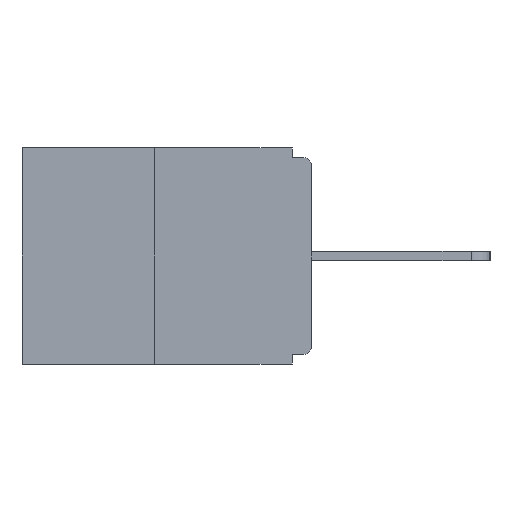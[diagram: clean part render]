
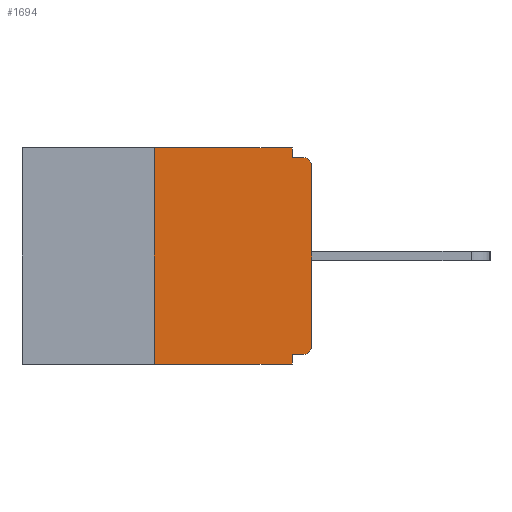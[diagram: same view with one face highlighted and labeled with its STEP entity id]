
A CAD part, left-side view. The second image highlights one B-rep face of the part: STEP entity #1694.
In plain terms, the highlighted planar face has unit normal (-1, 0, 0).
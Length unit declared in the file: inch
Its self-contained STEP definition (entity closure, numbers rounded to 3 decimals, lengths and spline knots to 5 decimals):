
#20 = CARTESIAN_POINT ( 'NONE',  ( 0., 0.46, 0. ) ) ;
#141 = CARTESIAN_POINT ( 'NONE',  ( 0., 0.015, -0.015 ) ) ;
#284 = CARTESIAN_POINT ( 'NONE',  ( 0., 0.031, 0. ) ) ;
#292 = LINE ( 'NONE', #13787, #13324 ) ;
#404 = EDGE_CURVE ( 'NONE', #16049, #15028, #6335, .T. ) ;
#788 = VERTEX_POINT ( 'NONE', #22123 ) ;
#1146 = VERTEX_POINT ( 'NONE', #5849 ) ;
#1694 = ADVANCED_FACE ( 'NONE', ( #17215 ), #3090, .F. ) ;
#1705 = VERTEX_POINT ( 'NONE', #16622 ) ;
#1894 = DIRECTION ( 'NONE',  ( 0., 0., -1. ) ) ;
#1922 = DIRECTION ( 'NONE',  ( -1., 0., 0. ) ) ;
#1966 = CARTESIAN_POINT ( 'NONE',  ( 0., 0.015, -0.03 ) ) ;
#2034 = EDGE_LOOP ( 'NONE', ( #8245, #4088, #13419, #9899, #2703, #16720, #3263, #17258, #22466, #19422 ) ) ;
#2648 = VERTEX_POINT ( 'NONE', #16496 ) ;
#2703 = ORIENTED_EDGE ( 'NONE', *, *, #9752, .F. ) ;
#3090 = PLANE ( 'NONE',  #18814 ) ;
#3263 = ORIENTED_EDGE ( 'NONE', *, *, #7796, .T. ) ;
#3947 = CARTESIAN_POINT ( 'NONE',  ( 0., 0., 0. ) ) ;
#3975 = DIRECTION ( 'NONE',  ( 0., 0., 1. ) ) ;
#4088 = ORIENTED_EDGE ( 'NONE', *, *, #10374, .F. ) ;
#4287 = VERTEX_POINT ( 'NONE', #141 ) ;
#4296 = LINE ( 'NONE', #3947, #18491 ) ;
#5050 = DIRECTION ( 'NONE',  ( 0., 0., -1. ) ) ;
#5373 = VECTOR ( 'NONE', #11786, 39.37008 ) ;
#5708 = CARTESIAN_POINT ( 'NONE',  ( 0., 0., -0.313 ) ) ;
#5849 = CARTESIAN_POINT ( 'NONE',  ( 0., 0.25, 0. ) ) ;
#5916 = LINE ( 'NONE', #10039, #5373 ) ;
#6121 = CARTESIAN_POINT ( 'NONE',  ( 0., 0., -0.015 ) ) ;
#6335 = CIRCLE ( 'NONE', #11204, 0.015 ) ;
#6812 = LINE ( 'NONE', #12746, #19632 ) ;
#6883 = LINE ( 'NONE', #20, #20272 ) ;
#7126 = VERTEX_POINT ( 'NONE', #11226 ) ;
#7226 = DIRECTION ( 'NONE',  ( -1., 0., 0. ) ) ;
#7796 = EDGE_CURVE ( 'NONE', #15028, #2648, #4296, .T. ) ;
#7945 = EDGE_CURVE ( 'NONE', #2648, #4287, #10362, .T. ) ;
#8245 = ORIENTED_EDGE ( 'NONE', *, *, #21274, .F. ) ;
#9752 = EDGE_CURVE ( 'NONE', #16049, #788, #6812, .T. ) ;
#9899 = ORIENTED_EDGE ( 'NONE', *, *, #10692, .F. ) ;
#10039 = CARTESIAN_POINT ( 'NONE',  ( 0., 0.031, 0. ) ) ;
#10362 = CIRCLE ( 'NONE', #14993, 0.015 ) ;
#10374 = EDGE_CURVE ( 'NONE', #1705, #1146, #16380, .T. ) ;
#10436 = VERTEX_POINT ( 'NONE', #18266 ) ;
#10692 = EDGE_CURVE ( 'NONE', #788, #10436, #292, .T. ) ;
#10855 = EDGE_CURVE ( 'NONE', #16241, #7126, #5916, .T. ) ;
#11204 = AXIS2_PLACEMENT_3D ( 'NONE', #16271, #7226, #11747 ) ;
#11226 = CARTESIAN_POINT ( 'NONE',  ( 0., 0.031, -0.015 ) ) ;
#11747 = DIRECTION ( 'NONE',  ( 0., 0., -1. ) ) ;
#11786 = DIRECTION ( 'NONE',  ( 0., 0., -1. ) ) ;
#12746 = CARTESIAN_POINT ( 'NONE',  ( 0., 0., -0.328 ) ) ;
#12875 = EDGE_CURVE ( 'NONE', #1705, #10436, #13781, .T. ) ;
#13324 = VECTOR ( 'NONE', #5050, 39.37008 ) ;
#13419 = ORIENTED_EDGE ( 'NONE', *, *, #12875, .T. ) ;
#13570 = VECTOR ( 'NONE', #16618, 39.37008 ) ;
#13781 = LINE ( 'NONE', #21096, #17857 ) ;
#13787 = CARTESIAN_POINT ( 'NONE',  ( 0., 0.031, -0.343 ) ) ;
#14516 = DIRECTION ( 'NONE',  ( 0., 1., 0. ) ) ;
#14660 = CARTESIAN_POINT ( 'NONE',  ( 0., 0.25, 0. ) ) ;
#14993 = AXIS2_PLACEMENT_3D ( 'NONE', #1966, #1922, #1894 ) ;
#15028 = VERTEX_POINT ( 'NONE', #5708 ) ;
#15846 = VECTOR ( 'NONE', #16414, 39.37008 ) ;
#16049 = VERTEX_POINT ( 'NONE', #22650 ) ;
#16241 = VERTEX_POINT ( 'NONE', #284 ) ;
#16271 = CARTESIAN_POINT ( 'NONE',  ( 0., 0.015, -0.313 ) ) ;
#16380 = LINE ( 'NONE', #14660, #15846 ) ;
#16414 = DIRECTION ( 'NONE',  ( 0., 0., 1. ) ) ;
#16496 = CARTESIAN_POINT ( 'NONE',  ( 0., 0., -0.03 ) ) ;
#16618 = DIRECTION ( 'NONE',  ( 0., -1., 0. ) ) ;
#16622 = CARTESIAN_POINT ( 'NONE',  ( 0., 0.25, -0.343 ) ) ;
#16720 = ORIENTED_EDGE ( 'NONE', *, *, #404, .T. ) ;
#17215 = FACE_OUTER_BOUND ( 'NONE', #2034, .T. ) ;
#17258 = ORIENTED_EDGE ( 'NONE', *, *, #7945, .T. ) ;
#17857 = VECTOR ( 'NONE', #22862, 39.37008 ) ;
#18266 = CARTESIAN_POINT ( 'NONE',  ( 0., 0.031, -0.343 ) ) ;
#18491 = VECTOR ( 'NONE', #3975, 39.37008 ) ;
#18814 = AXIS2_PLACEMENT_3D ( 'NONE', #22179, #22033, #18933 ) ;
#18933 = DIRECTION ( 'NONE',  ( 0., 0., -1. ) ) ;
#19422 = ORIENTED_EDGE ( 'NONE', *, *, #10855, .F. ) ;
#19432 = DIRECTION ( 'NONE',  ( 0., -1., 0. ) ) ;
#19632 = VECTOR ( 'NONE', #14516, 39.37008 ) ;
#20272 = VECTOR ( 'NONE', #19432, 39.37008 ) ;
#21096 = CARTESIAN_POINT ( 'NONE',  ( 0., 0.46, -0.343 ) ) ;
#21274 = EDGE_CURVE ( 'NONE', #1146, #16241, #6883, .T. ) ;
#22033 = DIRECTION ( 'NONE',  ( 1., 0., 0. ) ) ;
#22109 = EDGE_CURVE ( 'NONE', #7126, #4287, #22483, .T. ) ;
#22123 = CARTESIAN_POINT ( 'NONE',  ( 0., 0.031, -0.328 ) ) ;
#22179 = CARTESIAN_POINT ( 'NONE',  ( 0., 0.46, 0. ) ) ;
#22466 = ORIENTED_EDGE ( 'NONE', *, *, #22109, .F. ) ;
#22483 = LINE ( 'NONE', #6121, #13570 ) ;
#22650 = CARTESIAN_POINT ( 'NONE',  ( 0., 0.015, -0.328 ) ) ;
#22862 = DIRECTION ( 'NONE',  ( 0., -1., 0. ) ) ;
